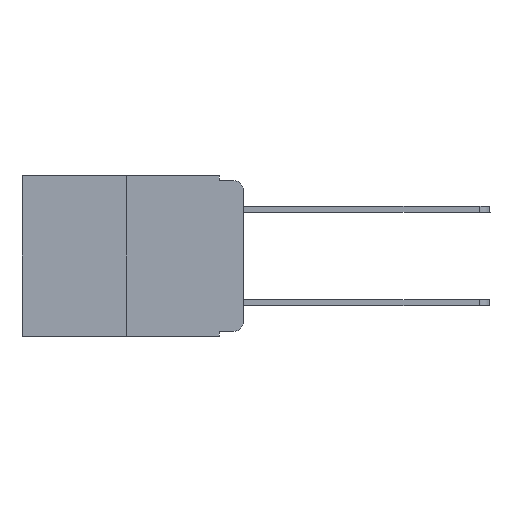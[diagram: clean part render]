
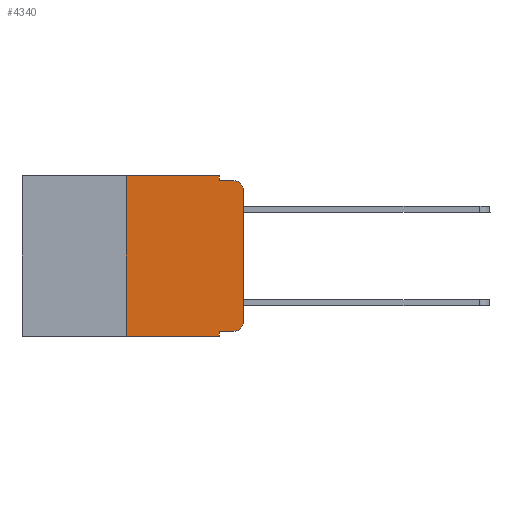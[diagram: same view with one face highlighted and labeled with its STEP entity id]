
A CAD part, left-side view. The second image highlights one B-rep face of the part: STEP entity #4340.
In plain terms, the highlighted planar face has unit normal (-1, 0, 0).
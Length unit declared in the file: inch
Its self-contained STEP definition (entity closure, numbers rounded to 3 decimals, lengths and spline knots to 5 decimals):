
#137 = CARTESIAN_POINT ( 'NONE',  ( 0., 0.02, -0.313 ) ) ;
#154 = DIRECTION ( 'NONE',  ( 0., 0., 1. ) ) ;
#540 = VERTEX_POINT ( 'NONE', #19029 ) ;
#795 = LINE ( 'NONE', #18921, #11975 ) ;
#863 = DIRECTION ( 'NONE',  ( 0., -1., 0. ) ) ;
#1189 = CARTESIAN_POINT ( 'NONE',  ( 0., 0., 0. ) ) ;
#1639 = DIRECTION ( 'NONE',  ( 0., 0., -1. ) ) ;
#1827 = CARTESIAN_POINT ( 'NONE',  ( 0., 0.473, 0. ) ) ;
#1979 = ORIENTED_EDGE ( 'NONE', *, *, #17092, .F. ) ;
#2041 = CARTESIAN_POINT ( 'NONE',  ( 0., 0.02, -0.333 ) ) ;
#2975 = EDGE_CURVE ( 'NONE', #7564, #3407, #17598, .T. ) ;
#3249 = EDGE_CURVE ( 'NONE', #8239, #8673, #795, .T. ) ;
#3407 = VERTEX_POINT ( 'NONE', #17470 ) ;
#3550 = CARTESIAN_POINT ( 'NONE',  ( 0., 0.051, 0. ) ) ;
#3591 = EDGE_CURVE ( 'NONE', #8673, #7564, #9457, .T. ) ;
#4340 = ADVANCED_FACE ( 'NONE', ( #19771 ), #5266, .F. ) ;
#4857 = CARTESIAN_POINT ( 'NONE',  ( 0., 0.051, -0.01 ) ) ;
#5245 = DIRECTION ( 'NONE',  ( -1., 0., 0. ) ) ;
#5266 = PLANE ( 'NONE',  #20115 ) ;
#5308 = ORIENTED_EDGE ( 'NONE', *, *, #2975, .F. ) ;
#5867 = EDGE_CURVE ( 'NONE', #22008, #10581, #19150, .T. ) ;
#6864 = ORIENTED_EDGE ( 'NONE', *, *, #20382, .T. ) ;
#7087 = AXIS2_PLACEMENT_3D ( 'NONE', #137, #5245, #1639 ) ;
#7564 = VERTEX_POINT ( 'NONE', #15390 ) ;
#8239 = VERTEX_POINT ( 'NONE', #16408 ) ;
#8350 = LINE ( 'NONE', #1189, #10841 ) ;
#8673 = VERTEX_POINT ( 'NONE', #16782 ) ;
#8864 = CARTESIAN_POINT ( 'NONE',  ( 0., 0.25, 0. ) ) ;
#8896 = CARTESIAN_POINT ( 'NONE',  ( 0., 0.051, -0.333 ) ) ;
#9073 = LINE ( 'NONE', #15377, #20837 ) ;
#9142 = ORIENTED_EDGE ( 'NONE', *, *, #17433, .T. ) ;
#9457 = LINE ( 'NONE', #3550, #18444 ) ;
#9707 = EDGE_CURVE ( 'NONE', #17383, #3407, #11393, .T. ) ;
#10186 = DIRECTION ( 'NONE',  ( 0., -1., 0. ) ) ;
#10303 = ORIENTED_EDGE ( 'NONE', *, *, #16212, .T. ) ;
#10581 = VERTEX_POINT ( 'NONE', #14329 ) ;
#10747 = VERTEX_POINT ( 'NONE', #18183 ) ;
#10841 = VECTOR ( 'NONE', #18820, 39.37008 ) ;
#11309 = AXIS2_PLACEMENT_3D ( 'NONE', #19937, #19859, #21635 ) ;
#11393 = CIRCLE ( 'NONE', #11309, 0.02 ) ;
#11842 = VERTEX_POINT ( 'NONE', #8896 ) ;
#11885 = EDGE_CURVE ( 'NONE', #11842, #10747, #17773, .T. ) ;
#11926 = ORIENTED_EDGE ( 'NONE', *, *, #3591, .F. ) ;
#11975 = VECTOR ( 'NONE', #10186, 39.37008 ) ;
#12112 = DIRECTION ( 'NONE',  ( 0., -1., 0. ) ) ;
#12437 = ORIENTED_EDGE ( 'NONE', *, *, #9707, .T. ) ;
#12986 = VECTOR ( 'NONE', #14585, 39.37008 ) ;
#13406 = VECTOR ( 'NONE', #12112, 39.37008 ) ;
#13976 = DIRECTION ( 'NONE',  ( 0., -1., 0. ) ) ;
#14329 = CARTESIAN_POINT ( 'NONE',  ( 0., 0., -0.313 ) ) ;
#14585 = DIRECTION ( 'NONE',  ( 0., 0., -1. ) ) ;
#15377 = CARTESIAN_POINT ( 'NONE',  ( 0., 0.473, -0.343 ) ) ;
#15390 = CARTESIAN_POINT ( 'NONE',  ( 0., 0.051, -0.01 ) ) ;
#15887 = DIRECTION ( 'NONE',  ( 0., 0., -1. ) ) ;
#16212 = EDGE_CURVE ( 'NONE', #11842, #22008, #22414, .T. ) ;
#16237 = CARTESIAN_POINT ( 'NONE',  ( 0., 0.051, 0. ) ) ;
#16408 = CARTESIAN_POINT ( 'NONE',  ( 0., 0.25, 0. ) ) ;
#16782 = CARTESIAN_POINT ( 'NONE',  ( 0., 0.051, 0. ) ) ;
#16963 = ORIENTED_EDGE ( 'NONE', *, *, #11885, .F. ) ;
#17092 = EDGE_CURVE ( 'NONE', #540, #8239, #17624, .T. ) ;
#17383 = VERTEX_POINT ( 'NONE', #18667 ) ;
#17433 = EDGE_CURVE ( 'NONE', #10581, #17383, #8350, .T. ) ;
#17470 = CARTESIAN_POINT ( 'NONE',  ( 0., 0.02, -0.01 ) ) ;
#17598 = LINE ( 'NONE', #4857, #19021 ) ;
#17624 = LINE ( 'NONE', #8864, #22365 ) ;
#17773 = LINE ( 'NONE', #16237, #12986 ) ;
#17879 = DIRECTION ( 'NONE',  ( 1., 0., 0. ) ) ;
#17931 = EDGE_LOOP ( 'NONE', ( #9142, #12437, #5308, #11926, #19963, #1979, #6864, #16963, #10303, #19088 ) ) ;
#18045 = DIRECTION ( 'NONE',  ( 0., 0., -1. ) ) ;
#18183 = CARTESIAN_POINT ( 'NONE',  ( 0., 0.051, -0.343 ) ) ;
#18444 = VECTOR ( 'NONE', #15887, 39.37008 ) ;
#18667 = CARTESIAN_POINT ( 'NONE',  ( 0., 0., -0.03 ) ) ;
#18820 = DIRECTION ( 'NONE',  ( 0., 0., 1. ) ) ;
#18921 = CARTESIAN_POINT ( 'NONE',  ( 0., 0.473, 0. ) ) ;
#19021 = VECTOR ( 'NONE', #13976, 39.37008 ) ;
#19029 = CARTESIAN_POINT ( 'NONE',  ( 0., 0.25, -0.343 ) ) ;
#19088 = ORIENTED_EDGE ( 'NONE', *, *, #5867, .T. ) ;
#19150 = CIRCLE ( 'NONE', #7087, 0.02 ) ;
#19771 = FACE_OUTER_BOUND ( 'NONE', #17931, .T. ) ;
#19859 = DIRECTION ( 'NONE',  ( -1., 0., 0. ) ) ;
#19937 = CARTESIAN_POINT ( 'NONE',  ( 0., 0.02, -0.03 ) ) ;
#19963 = ORIENTED_EDGE ( 'NONE', *, *, #3249, .F. ) ;
#20115 = AXIS2_PLACEMENT_3D ( 'NONE', #1827, #17879, #18045 ) ;
#20382 = EDGE_CURVE ( 'NONE', #540, #10747, #9073, .T. ) ;
#20837 = VECTOR ( 'NONE', #863, 39.37008 ) ;
#21363 = CARTESIAN_POINT ( 'NONE',  ( 0., 0.051, -0.333 ) ) ;
#21635 = DIRECTION ( 'NONE',  ( 0., 0., -1. ) ) ;
#22008 = VERTEX_POINT ( 'NONE', #2041 ) ;
#22365 = VECTOR ( 'NONE', #154, 39.37008 ) ;
#22414 = LINE ( 'NONE', #21363, #13406 ) ;
